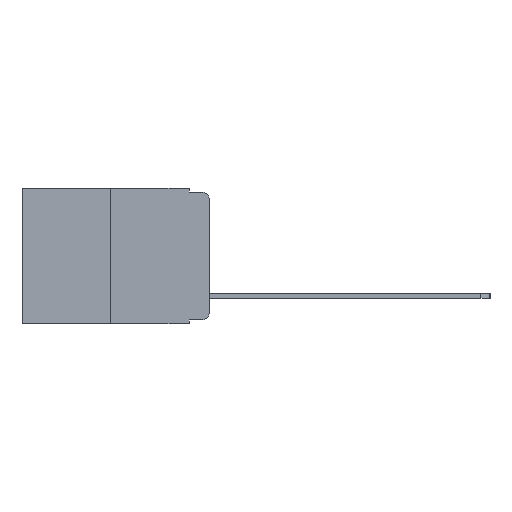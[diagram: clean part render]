
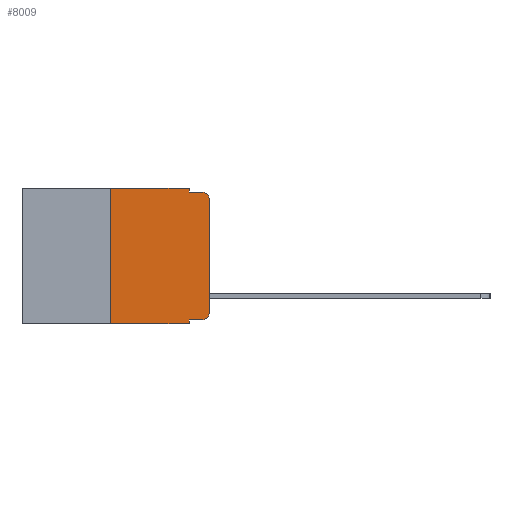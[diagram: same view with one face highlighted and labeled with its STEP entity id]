
A CAD part, left-side view. The second image highlights one B-rep face of the part: STEP entity #8009.
In plain terms, the highlighted planar face has unit normal (-1, 0, 0).
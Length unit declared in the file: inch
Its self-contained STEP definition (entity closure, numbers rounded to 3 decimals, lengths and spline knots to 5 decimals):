
#632 = EDGE_CURVE ( 'NONE', #2781, #9616, #16726, .T. ) ;
#974 = ORIENTED_EDGE ( 'NONE', *, *, #15195, .T. ) ;
#1034 = ORIENTED_EDGE ( 'NONE', *, *, #17693, .T. ) ;
#1091 = DIRECTION ( 'NONE',  ( 0., 0., -1. ) ) ;
#1914 = CARTESIAN_POINT ( 'NONE',  ( 0., 0.051, -0.333 ) ) ;
#1931 = LINE ( 'NONE', #11103, #5483 ) ;
#2435 = CARTESIAN_POINT ( 'NONE',  ( 0., 0.02, -0.333 ) ) ;
#2439 = VERTEX_POINT ( 'NONE', #14765 ) ;
#2723 = ORIENTED_EDGE ( 'NONE', *, *, #18562, .T. ) ;
#2781 = VERTEX_POINT ( 'NONE', #7021 ) ;
#2876 = VERTEX_POINT ( 'NONE', #4401 ) ;
#3100 = LINE ( 'NONE', #13767, #10464 ) ;
#3573 = CARTESIAN_POINT ( 'NONE',  ( 0., 0.02, -0.313 ) ) ;
#3673 = DIRECTION ( 'NONE',  ( 0., 0., -1. ) ) ;
#4041 = VERTEX_POINT ( 'NONE', #11921 ) ;
#4228 = VERTEX_POINT ( 'NONE', #6786 ) ;
#4267 = CARTESIAN_POINT ( 'NONE',  ( 0., 0.051, -0.01 ) ) ;
#4317 = ORIENTED_EDGE ( 'NONE', *, *, #6694, .F. ) ;
#4401 = CARTESIAN_POINT ( 'NONE',  ( 0., 0.051, 0. ) ) ;
#4508 = DIRECTION ( 'NONE',  ( 0., 0., -1. ) ) ;
#4597 = VERTEX_POINT ( 'NONE', #4611 ) ;
#4611 = CARTESIAN_POINT ( 'NONE',  ( 0., 0.25, 0. ) ) ;
#4740 = AXIS2_PLACEMENT_3D ( 'NONE', #18249, #9984, #1091 ) ;
#4932 = LINE ( 'NONE', #6569, #12622 ) ;
#5052 = ORIENTED_EDGE ( 'NONE', *, *, #9184, .F. ) ;
#5112 = DIRECTION ( 'NONE',  ( 0., 0., -1. ) ) ;
#5483 = VECTOR ( 'NONE', #12529, 39.37008 ) ;
#5743 = ORIENTED_EDGE ( 'NONE', *, *, #16208, .F. ) ;
#5931 = AXIS2_PLACEMENT_3D ( 'NONE', #7460, #13141, #4508 ) ;
#5947 = CIRCLE ( 'NONE', #18480, 0.02 ) ;
#6072 = EDGE_CURVE ( 'NONE', #18413, #4041, #1931, .T. ) ;
#6230 = LINE ( 'NONE', #13053, #9665 ) ;
#6319 = ORIENTED_EDGE ( 'NONE', *, *, #12329, .F. ) ;
#6396 = ORIENTED_EDGE ( 'NONE', *, *, #6072, .T. ) ;
#6514 = FACE_OUTER_BOUND ( 'NONE', #18081, .T. ) ;
#6519 = LINE ( 'NONE', #9426, #17285 ) ;
#6569 = CARTESIAN_POINT ( 'NONE',  ( 0., 0.25, 0. ) ) ;
#6694 = EDGE_CURVE ( 'NONE', #13065, #4228, #3100, .T. ) ;
#6786 = CARTESIAN_POINT ( 'NONE',  ( 0., 0.02, -0.01 ) ) ;
#7021 = CARTESIAN_POINT ( 'NONE',  ( 0., 0.051, -0.333 ) ) ;
#7325 = VECTOR ( 'NONE', #14003, 39.37008 ) ;
#7460 = CARTESIAN_POINT ( 'NONE',  ( 0., 0.473, 0. ) ) ;
#7483 = ORIENTED_EDGE ( 'NONE', *, *, #11737, .F. ) ;
#8009 = ADVANCED_FACE ( 'NONE', ( #6514 ), #11721, .F. ) ;
#8028 = DIRECTION ( 'NONE',  ( 0., 0., 1. ) ) ;
#8177 = CARTESIAN_POINT ( 'NONE',  ( 0., 0.25, -0.343 ) ) ;
#8874 = CARTESIAN_POINT ( 'NONE',  ( 0., 0.051, 0. ) ) ;
#9184 = EDGE_CURVE ( 'NONE', #2876, #13065, #16846, .T. ) ;
#9426 = CARTESIAN_POINT ( 'NONE',  ( 0., 0., 0. ) ) ;
#9616 = VERTEX_POINT ( 'NONE', #2435 ) ;
#9635 = DIRECTION ( 'NONE',  ( 0., -1., 0. ) ) ;
#9665 = VECTOR ( 'NONE', #14443, 39.37008 ) ;
#9837 = ORIENTED_EDGE ( 'NONE', *, *, #632, .T. ) ;
#9984 = DIRECTION ( 'NONE',  ( -1., 0., 0. ) ) ;
#10464 = VECTOR ( 'NONE', #9635, 39.37008 ) ;
#11103 = CARTESIAN_POINT ( 'NONE',  ( 0., 0.473, -0.343 ) ) ;
#11721 = PLANE ( 'NONE',  #5931 ) ;
#11737 = EDGE_CURVE ( 'NONE', #2781, #4041, #14821, .T. ) ;
#11921 = CARTESIAN_POINT ( 'NONE',  ( 0., 0.051, -0.343 ) ) ;
#12275 = CARTESIAN_POINT ( 'NONE',  ( 0., 0., -0.313 ) ) ;
#12329 = EDGE_CURVE ( 'NONE', #18413, #4597, #4932, .T. ) ;
#12332 = CARTESIAN_POINT ( 'NONE',  ( 0., 0.051, 0. ) ) ;
#12529 = DIRECTION ( 'NONE',  ( 0., -1., 0. ) ) ;
#12622 = VECTOR ( 'NONE', #17768, 39.37008 ) ;
#13053 = CARTESIAN_POINT ( 'NONE',  ( 0., 0.473, 0. ) ) ;
#13065 = VERTEX_POINT ( 'NONE', #4267 ) ;
#13086 = CIRCLE ( 'NONE', #4740, 0.02 ) ;
#13109 = DIRECTION ( 'NONE',  ( 0., 0., -1. ) ) ;
#13141 = DIRECTION ( 'NONE',  ( 1., 0., 0. ) ) ;
#13427 = VERTEX_POINT ( 'NONE', #12275 ) ;
#13610 = VECTOR ( 'NONE', #13109, 39.37008 ) ;
#13693 = DIRECTION ( 'NONE',  ( -1., 0., 0. ) ) ;
#13767 = CARTESIAN_POINT ( 'NONE',  ( 0., 0.051, -0.01 ) ) ;
#14003 = DIRECTION ( 'NONE',  ( 0., -1., 0. ) ) ;
#14443 = DIRECTION ( 'NONE',  ( 0., -1., 0. ) ) ;
#14765 = CARTESIAN_POINT ( 'NONE',  ( 0., 0., -0.03 ) ) ;
#14821 = LINE ( 'NONE', #12332, #17991 ) ;
#15195 = EDGE_CURVE ( 'NONE', #13427, #2439, #6519, .T. ) ;
#16208 = EDGE_CURVE ( 'NONE', #4597, #2876, #6230, .T. ) ;
#16726 = LINE ( 'NONE', #1914, #7325 ) ;
#16846 = LINE ( 'NONE', #8874, #13610 ) ;
#17285 = VECTOR ( 'NONE', #8028, 39.37008 ) ;
#17693 = EDGE_CURVE ( 'NONE', #9616, #13427, #5947, .T. ) ;
#17768 = DIRECTION ( 'NONE',  ( 0., 0., 1. ) ) ;
#17991 = VECTOR ( 'NONE', #3673, 39.37008 ) ;
#18081 = EDGE_LOOP ( 'NONE', ( #974, #2723, #4317, #5052, #5743, #6319, #6396, #7483, #9837, #1034 ) ) ;
#18249 = CARTESIAN_POINT ( 'NONE',  ( 0., 0.02, -0.03 ) ) ;
#18413 = VERTEX_POINT ( 'NONE', #8177 ) ;
#18480 = AXIS2_PLACEMENT_3D ( 'NONE', #3573, #13693, #5112 ) ;
#18562 = EDGE_CURVE ( 'NONE', #2439, #4228, #13086, .T. ) ;
